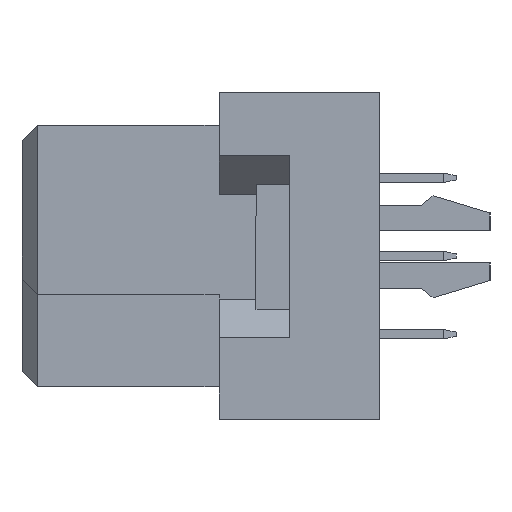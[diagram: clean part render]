
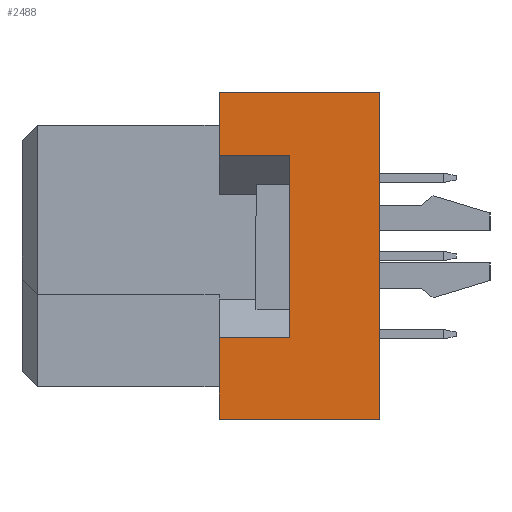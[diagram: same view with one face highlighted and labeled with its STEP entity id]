
A CAD part, left-side view. The second image highlights one B-rep face of the part: STEP entity #2488.
In plain terms, the highlighted planar face has unit normal (-1, 0, 0).
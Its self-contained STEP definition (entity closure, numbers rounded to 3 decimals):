
#474 = VECTOR ( 'NONE', #6007, 1000. ) ;
#512 = LINE ( 'NONE', #13989, #8203 ) ;
#890 = VECTOR ( 'NONE', #6756, 1000. ) ;
#1276 = EDGE_CURVE ( 'NONE', #8512, #6284, #7178, .T. ) ;
#1620 = CARTESIAN_POINT ( 'NONE',  ( -27.5, -6.4, -5.3 ) ) ;
#1631 = VECTOR ( 'NONE', #16558, 1000. ) ;
#1858 = CARTESIAN_POINT ( 'NONE',  ( -27.5, -8.7, 3.25 ) ) ;
#1874 = VERTEX_POINT ( 'NONE', #9382 ) ;
#1962 = VECTOR ( 'NONE', #20042, 1000. ) ;
#2326 = LINE ( 'NONE', #20481, #15874 ) ;
#2488 = ADVANCED_FACE ( 'NONE', ( #8657 ), #19554, .T. ) ;
#3210 = LINE ( 'NONE', #1620, #890 ) ;
#3752 = EDGE_CURVE ( 'NONE', #17914, #8084, #2326, .T. ) ;
#3804 = ORIENTED_EDGE ( 'NONE', *, *, #4063, .F. ) ;
#3926 = AXIS2_PLACEMENT_3D ( 'NONE', #15438, #21225, #6980 ) ;
#3992 = DIRECTION ( 'NONE',  ( 0., 1., 0. ) ) ;
#4013 = CARTESIAN_POINT ( 'NONE',  ( -27.5, -11.6, -5.3 ) ) ;
#4063 = EDGE_CURVE ( 'NONE', #6928, #1874, #3210, .T. ) ;
#4118 = DIRECTION ( 'NONE',  ( 0., 1., 0. ) ) ;
#4757 = CARTESIAN_POINT ( 'NONE',  ( -27.5, -11.6, 5.3 ) ) ;
#5082 = EDGE_LOOP ( 'NONE', ( #18132, #3804, #17361, #12925, #21830, #11255, #11147, #7302 ) ) ;
#5777 = CARTESIAN_POINT ( 'NONE',  ( -27.5, -8.7, 3.25 ) ) ;
#5868 = EDGE_CURVE ( 'NONE', #21792, #6928, #19604, .T. ) ;
#6007 = DIRECTION ( 'NONE',  ( 0., 1., 0. ) ) ;
#6284 = VERTEX_POINT ( 'NONE', #1858 ) ;
#6506 = EDGE_CURVE ( 'NONE', #8512, #1874, #9553, .T. ) ;
#6756 = DIRECTION ( 'NONE',  ( 0., 0., 1. ) ) ;
#6928 = VERTEX_POINT ( 'NONE', #18114 ) ;
#6980 = DIRECTION ( 'NONE',  ( 0., 0., 1. ) ) ;
#7178 = LINE ( 'NONE', #8970, #21468 ) ;
#7302 = ORIENTED_EDGE ( 'NONE', *, *, #1276, .F. ) ;
#7672 = EDGE_CURVE ( 'NONE', #16807, #8084, #512, .T. ) ;
#8084 = VERTEX_POINT ( 'NONE', #17449 ) ;
#8203 = VECTOR ( 'NONE', #3992, 1000. ) ;
#8512 = VERTEX_POINT ( 'NONE', #12271 ) ;
#8657 = FACE_OUTER_BOUND ( 'NONE', #5082, .T. ) ;
#8970 = CARTESIAN_POINT ( 'NONE',  ( -27.5, -8.7, -2.65 ) ) ;
#9382 = CARTESIAN_POINT ( 'NONE',  ( -27.5, -6.4, -2.65 ) ) ;
#9553 = LINE ( 'NONE', #16452, #1631 ) ;
#11147 = ORIENTED_EDGE ( 'NONE', *, *, #20287, .F. ) ;
#11255 = ORIENTED_EDGE ( 'NONE', *, *, #3752, .F. ) ;
#11348 = LINE ( 'NONE', #15009, #1962 ) ;
#12271 = CARTESIAN_POINT ( 'NONE',  ( -27.5, -8.7, -2.65 ) ) ;
#12925 = ORIENTED_EDGE ( 'NONE', *, *, #21808, .T. ) ;
#13989 = CARTESIAN_POINT ( 'NONE',  ( -27.5, -11.6, 5.3 ) ) ;
#14335 = LINE ( 'NONE', #5777, #474 ) ;
#14403 = VECTOR ( 'NONE', #4118, 1000. ) ;
#15009 = CARTESIAN_POINT ( 'NONE',  ( -27.5, -11.6, 5.3 ) ) ;
#15438 = CARTESIAN_POINT ( 'NONE',  ( -27.5, -11.6, 5.3 ) ) ;
#15874 = VECTOR ( 'NONE', #15890, 1000. ) ;
#15890 = DIRECTION ( 'NONE',  ( 0., 0., 1. ) ) ;
#16452 = CARTESIAN_POINT ( 'NONE',  ( -27.5, -8.7, -2.65 ) ) ;
#16558 = DIRECTION ( 'NONE',  ( 0., 1., 0. ) ) ;
#16807 = VERTEX_POINT ( 'NONE', #4757 ) ;
#17361 = ORIENTED_EDGE ( 'NONE', *, *, #5868, .F. ) ;
#17449 = CARTESIAN_POINT ( 'NONE',  ( -27.5, -6.4, 5.3 ) ) ;
#17914 = VERTEX_POINT ( 'NONE', #20524 ) ;
#18114 = CARTESIAN_POINT ( 'NONE',  ( -27.5, -6.4, -5.3 ) ) ;
#18132 = ORIENTED_EDGE ( 'NONE', *, *, #6506, .T. ) ;
#19323 = DIRECTION ( 'NONE',  ( 0., 0., 1. ) ) ;
#19554 = PLANE ( 'NONE',  #3926 ) ;
#19604 = LINE ( 'NONE', #4013, #14403 ) ;
#20042 = DIRECTION ( 'NONE',  ( 0., 0., 1. ) ) ;
#20287 = EDGE_CURVE ( 'NONE', #6284, #17914, #14335, .T. ) ;
#20481 = CARTESIAN_POINT ( 'NONE',  ( -27.5, -6.4, -5.3 ) ) ;
#20524 = CARTESIAN_POINT ( 'NONE',  ( -27.5, -6.4, 3.25 ) ) ;
#21225 = DIRECTION ( 'NONE',  ( -1., 0., 0. ) ) ;
#21468 = VECTOR ( 'NONE', #19323, 1000. ) ;
#21792 = VERTEX_POINT ( 'NONE', #21816 ) ;
#21808 = EDGE_CURVE ( 'NONE', #21792, #16807, #11348, .T. ) ;
#21816 = CARTESIAN_POINT ( 'NONE',  ( -27.5, -11.6, -5.3 ) ) ;
#21830 = ORIENTED_EDGE ( 'NONE', *, *, #7672, .T. ) ;
